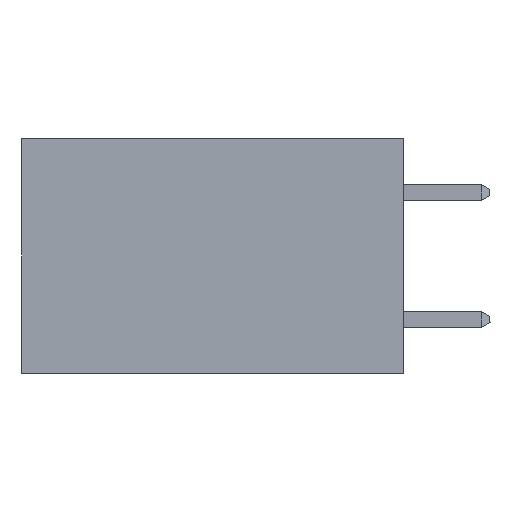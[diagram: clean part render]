
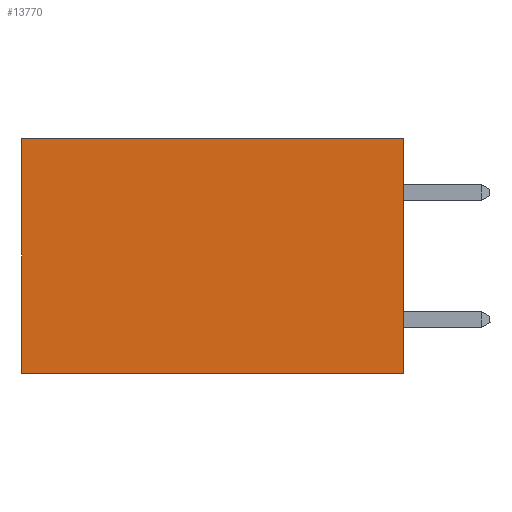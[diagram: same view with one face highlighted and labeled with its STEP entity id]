
A CAD part, left-side view. The second image highlights one B-rep face of the part: STEP entity #13770.
In plain terms, the highlighted planar face has unit normal (-1, 0, 0).
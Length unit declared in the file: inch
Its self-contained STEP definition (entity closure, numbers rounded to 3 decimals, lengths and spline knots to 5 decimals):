
#917 = LINE ( 'NONE', #2795, #8548 ) ;
#1543 = CARTESIAN_POINT ( 'NONE',  ( 0.2875, 0., -0.37 ) ) ;
#1941 = VERTEX_POINT ( 'NONE', #10457 ) ;
#2795 = CARTESIAN_POINT ( 'NONE',  ( 0.2875, 0., 0. ) ) ;
#2826 = FACE_OUTER_BOUND ( 'NONE', #5028, .T. ) ;
#2920 = CARTESIAN_POINT ( 'NONE',  ( 0.2875, 0., 0. ) ) ;
#2988 = LINE ( 'NONE', #14652, #15183 ) ;
#3340 = CARTESIAN_POINT ( 'NONE',  ( 0.2875, 0.6, 0. ) ) ;
#3389 = VERTEX_POINT ( 'NONE', #9385 ) ;
#3729 = ORIENTED_EDGE ( 'NONE', *, *, #8420, .T. ) ;
#4967 = PLANE ( 'NONE',  #10831 ) ;
#5015 = DIRECTION ( 'NONE',  ( 0., 0., -1. ) ) ;
#5016 = LINE ( 'NONE', #2920, #14360 ) ;
#5028 = EDGE_LOOP ( 'NONE', ( #3729, #13261, #9212, #13900 ) ) ;
#5137 = VECTOR ( 'NONE', #7529, 39.37008 ) ;
#5903 = LINE ( 'NONE', #1543, #5137 ) ;
#7529 = DIRECTION ( 'NONE',  ( 0., 1., 0. ) ) ;
#7833 = EDGE_CURVE ( 'NONE', #9433, #3389, #917, .T. ) ;
#8420 = EDGE_CURVE ( 'NONE', #14543, #1941, #2988, .T. ) ;
#8548 = VECTOR ( 'NONE', #14829, 39.37008 ) ;
#9212 = ORIENTED_EDGE ( 'NONE', *, *, #7833, .F. ) ;
#9385 = CARTESIAN_POINT ( 'NONE',  ( 0.2875, 0., -0.37 ) ) ;
#9433 = VERTEX_POINT ( 'NONE', #12223 ) ;
#10457 = CARTESIAN_POINT ( 'NONE',  ( 0.2875, 0.6, -0.37 ) ) ;
#10659 = EDGE_CURVE ( 'NONE', #9433, #14543, #5016, .T. ) ;
#10831 = AXIS2_PLACEMENT_3D ( 'NONE', #13390, #11174, #5015 ) ;
#11174 = DIRECTION ( 'NONE',  ( 1., 0., 0. ) ) ;
#11473 = DIRECTION ( 'NONE',  ( 0., 1., 0. ) ) ;
#12223 = CARTESIAN_POINT ( 'NONE',  ( 0.2875, 0., 0. ) ) ;
#12704 = EDGE_CURVE ( 'NONE', #3389, #1941, #5903, .T. ) ;
#13261 = ORIENTED_EDGE ( 'NONE', *, *, #12704, .F. ) ;
#13328 = DIRECTION ( 'NONE',  ( 0., 0., -1. ) ) ;
#13390 = CARTESIAN_POINT ( 'NONE',  ( 0.2875, 0., 0. ) ) ;
#13770 = ADVANCED_FACE ( 'NONE', ( #2826 ), #4967, .F. ) ;
#13900 = ORIENTED_EDGE ( 'NONE', *, *, #10659, .T. ) ;
#14360 = VECTOR ( 'NONE', #11473, 39.37008 ) ;
#14543 = VERTEX_POINT ( 'NONE', #3340 ) ;
#14652 = CARTESIAN_POINT ( 'NONE',  ( 0.2875, 0.6, 0. ) ) ;
#14829 = DIRECTION ( 'NONE',  ( 0., 0., -1. ) ) ;
#15183 = VECTOR ( 'NONE', #13328, 39.37008 ) ;
